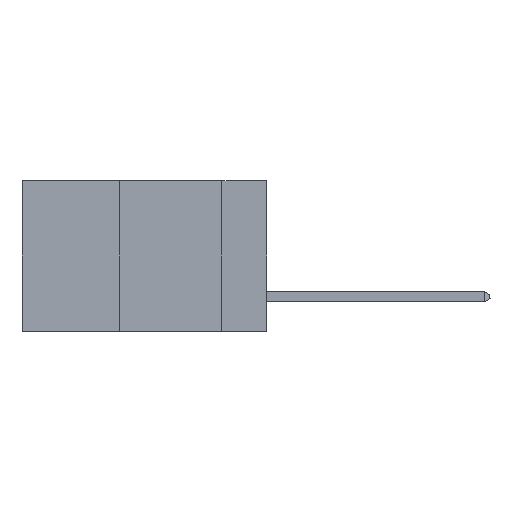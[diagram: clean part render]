
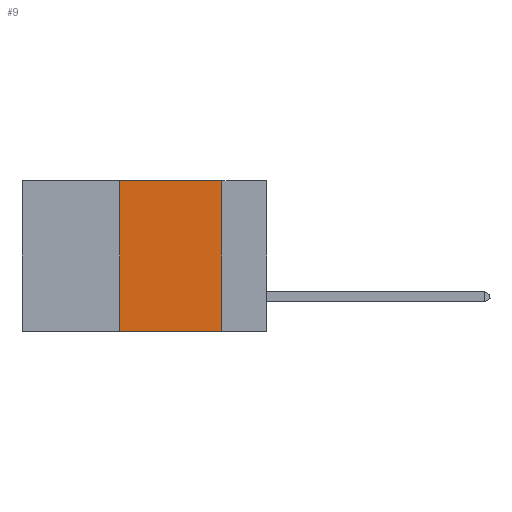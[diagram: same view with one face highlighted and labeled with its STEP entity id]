
A CAD part, left-side view. The second image highlights one B-rep face of the part: STEP entity #9.
In plain terms, the highlighted planar face has unit normal (-1, 0, 0).
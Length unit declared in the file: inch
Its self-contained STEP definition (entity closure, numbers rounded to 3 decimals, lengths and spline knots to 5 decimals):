
#9 = ADVANCED_FACE ( 'NONE', ( #13130 ), #3269, .F. ) ;
#254 = ORIENTED_EDGE ( 'NONE', *, *, #1208, .F. ) ;
#839 = VECTOR ( 'NONE', #1837, 39.37008 ) ;
#1208 = EDGE_CURVE ( 'NONE', #14636, #9969, #11432, .T. ) ;
#1363 = DIRECTION ( 'NONE',  ( 0., -1., 0. ) ) ;
#1837 = DIRECTION ( 'NONE',  ( 0., 0., -1. ) ) ;
#1913 = DIRECTION ( 'NONE',  ( 1., 0., 0. ) ) ;
#2265 = DIRECTION ( 'NONE',  ( 0., -1., 0. ) ) ;
#2349 = LINE ( 'NONE', #10461, #10604 ) ;
#3253 = CARTESIAN_POINT ( 'NONE',  ( 0., 0.11, 0. ) ) ;
#3269 = PLANE ( 'NONE',  #5745 ) ;
#3319 = ORIENTED_EDGE ( 'NONE', *, *, #12380, .T. ) ;
#3437 = EDGE_CURVE ( 'NONE', #3929, #6959, #2349, .T. ) ;
#3526 = CARTESIAN_POINT ( 'NONE',  ( 0., 0.6, 0. ) ) ;
#3929 = VERTEX_POINT ( 'NONE', #7470 ) ;
#4790 = VECTOR ( 'NONE', #2265, 39.37008 ) ;
#5082 = DIRECTION ( 'NONE',  ( 0., 0., 1. ) ) ;
#5161 = LINE ( 'NONE', #5381, #9221 ) ;
#5381 = CARTESIAN_POINT ( 'NONE',  ( 0., 0.6, -0.37 ) ) ;
#5564 = CARTESIAN_POINT ( 'NONE',  ( 0., 0.11, 0. ) ) ;
#5745 = AXIS2_PLACEMENT_3D ( 'NONE', #10085, #1913, #7368 ) ;
#6959 = VERTEX_POINT ( 'NONE', #13906 ) ;
#7368 = DIRECTION ( 'NONE',  ( 0., 0., -1. ) ) ;
#7470 = CARTESIAN_POINT ( 'NONE',  ( 0., 0.36, -0.37 ) ) ;
#7554 = LINE ( 'NONE', #3526, #4790 ) ;
#9221 = VECTOR ( 'NONE', #1363, 39.37008 ) ;
#9421 = EDGE_LOOP ( 'NONE', ( #254, #11877, #16331, #3319 ) ) ;
#9969 = VERTEX_POINT ( 'NONE', #10145 ) ;
#10085 = CARTESIAN_POINT ( 'NONE',  ( 0., 0.6, 0. ) ) ;
#10145 = CARTESIAN_POINT ( 'NONE',  ( 0., 0.11, -0.37 ) ) ;
#10461 = CARTESIAN_POINT ( 'NONE',  ( 0., 0.36, 0. ) ) ;
#10604 = VECTOR ( 'NONE', #5082, 39.37008 ) ;
#11432 = LINE ( 'NONE', #3253, #839 ) ;
#11877 = ORIENTED_EDGE ( 'NONE', *, *, #14342, .F. ) ;
#12380 = EDGE_CURVE ( 'NONE', #3929, #9969, #5161, .T. ) ;
#13130 = FACE_OUTER_BOUND ( 'NONE', #9421, .T. ) ;
#13906 = CARTESIAN_POINT ( 'NONE',  ( 0., 0.36, 0. ) ) ;
#14342 = EDGE_CURVE ( 'NONE', #6959, #14636, #7554, .T. ) ;
#14636 = VERTEX_POINT ( 'NONE', #5564 ) ;
#16331 = ORIENTED_EDGE ( 'NONE', *, *, #3437, .F. ) ;
